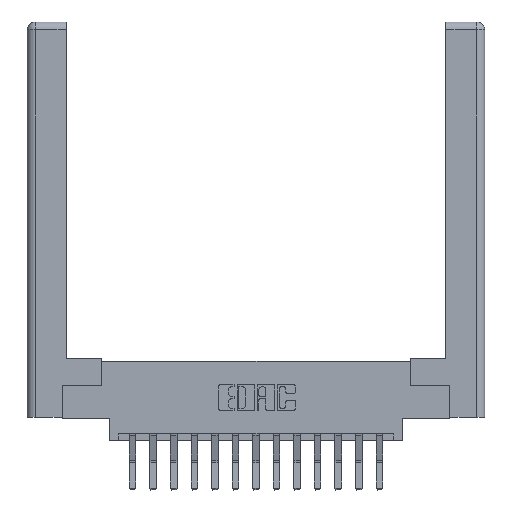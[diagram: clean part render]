
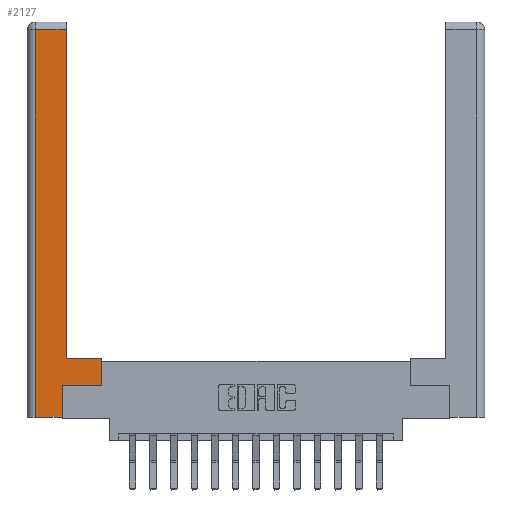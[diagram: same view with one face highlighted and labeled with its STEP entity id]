
A CAD part, top view. The second image highlights one B-rep face of the part: STEP entity #2127.
In plain terms, the highlighted planar face has unit normal (0, 0, 1).
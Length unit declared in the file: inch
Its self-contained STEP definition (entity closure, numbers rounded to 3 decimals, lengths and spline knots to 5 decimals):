
#1 = VECTOR ( 'NONE', #6524, 39.37008 ) ;
#176 = LINE ( 'NONE', #9322, #4261 ) ;
#615 = VERTEX_POINT ( 'NONE', #15131 ) ;
#640 = EDGE_CURVE ( 'NONE', #4127, #615, #4066, .T. ) ;
#830 = ORIENTED_EDGE ( 'NONE', *, *, #15073, .T. ) ;
#904 = CARTESIAN_POINT ( 'NONE',  ( 0., 0., 0. ) ) ;
#1306 = DIRECTION ( 'NONE',  ( 1., 0., 0. ) ) ;
#1787 = LINE ( 'NONE', #5879, #7243 ) ;
#2127 = ADVANCED_FACE ( 'NONE', ( #13701 ), #5015, .F. ) ;
#2202 = EDGE_CURVE ( 'NONE', #4471, #12927, #1787, .T. ) ;
#2537 = EDGE_LOOP ( 'NONE', ( #14064, #10161, #830, #11777, #7484, #6974, #5927, #4279 ) ) ;
#2657 = AXIS2_PLACEMENT_3D ( 'NONE', #904, #6328, #9095 ) ;
#2907 = VERTEX_POINT ( 'NONE', #4724 ) ;
#3094 = DIRECTION ( 'NONE',  ( -1., 0., 0. ) ) ;
#3812 = CARTESIAN_POINT ( 'NONE',  ( 0.265, 0., 0. ) ) ;
#4066 = LINE ( 'NONE', #14343, #1 ) ;
#4127 = VERTEX_POINT ( 'NONE', #9582 ) ;
#4261 = VECTOR ( 'NONE', #5508, 39.37008 ) ;
#4279 = ORIENTED_EDGE ( 'NONE', *, *, #16211, .T. ) ;
#4471 = VERTEX_POINT ( 'NONE', #13369 ) ;
#4724 = CARTESIAN_POINT ( 'NONE',  ( 0.565, 0.245, 0. ) ) ;
#4844 = DIRECTION ( 'NONE',  ( -1., 0., 0. ) ) ;
#5015 = PLANE ( 'NONE',  #2657 ) ;
#5061 = CARTESIAN_POINT ( 'NONE',  ( 0.0615, 2.94, 0. ) ) ;
#5339 = VECTOR ( 'NONE', #8675, 39.37008 ) ;
#5508 = DIRECTION ( 'NONE',  ( 0., 1., 0. ) ) ;
#5879 = CARTESIAN_POINT ( 'NONE',  ( 0.295, 3., 0. ) ) ;
#5902 = VECTOR ( 'NONE', #7099, 39.37008 ) ;
#5927 = ORIENTED_EDGE ( 'NONE', *, *, #5997, .T. ) ;
#5997 = EDGE_CURVE ( 'NONE', #2907, #6063, #176, .T. ) ;
#6063 = VERTEX_POINT ( 'NONE', #10544 ) ;
#6232 = CARTESIAN_POINT ( 'NONE',  ( 0.0615, 0., 0. ) ) ;
#6328 = DIRECTION ( 'NONE',  ( 0., 0., -1. ) ) ;
#6524 = DIRECTION ( 'NONE',  ( 0., 1., 0. ) ) ;
#6561 = VERTEX_POINT ( 'NONE', #5061 ) ;
#6716 = VECTOR ( 'NONE', #3094, 39.37008 ) ;
#6974 = ORIENTED_EDGE ( 'NONE', *, *, #9352, .T. ) ;
#7099 = DIRECTION ( 'NONE',  ( 0., -1., 0. ) ) ;
#7243 = VECTOR ( 'NONE', #9892, 39.37008 ) ;
#7256 = CARTESIAN_POINT ( 'NONE',  ( 0.565, 0.245, 0. ) ) ;
#7484 = ORIENTED_EDGE ( 'NONE', *, *, #640, .T. ) ;
#8583 = LINE ( 'NONE', #12562, #8961 ) ;
#8664 = VECTOR ( 'NONE', #1306, 39.37008 ) ;
#8675 = DIRECTION ( 'NONE',  ( 1., 0., 0. ) ) ;
#8795 = LINE ( 'NONE', #7256, #5339 ) ;
#8961 = VECTOR ( 'NONE', #4844, 39.37008 ) ;
#9095 = DIRECTION ( 'NONE',  ( -1., 0., 0. ) ) ;
#9322 = CARTESIAN_POINT ( 'NONE',  ( 0.565, 0.45, 0. ) ) ;
#9337 = LINE ( 'NONE', #10840, #5902 ) ;
#9352 = EDGE_CURVE ( 'NONE', #615, #2907, #8795, .T. ) ;
#9582 = CARTESIAN_POINT ( 'NONE',  ( 0.265, 0., 0. ) ) ;
#9892 = DIRECTION ( 'NONE',  ( 0., 1., 0. ) ) ;
#10161 = ORIENTED_EDGE ( 'NONE', *, *, #13758, .T. ) ;
#10499 = EDGE_CURVE ( 'NONE', #13332, #4127, #12892, .T. ) ;
#10544 = CARTESIAN_POINT ( 'NONE',  ( 0.565, 0.45, 0. ) ) ;
#10574 = LINE ( 'NONE', #13539, #6716 ) ;
#10840 = CARTESIAN_POINT ( 'NONE',  ( 0.0615, 0., 0. ) ) ;
#11777 = ORIENTED_EDGE ( 'NONE', *, *, #10499, .T. ) ;
#11831 = CARTESIAN_POINT ( 'NONE',  ( 0.295, 2.94, 0. ) ) ;
#12562 = CARTESIAN_POINT ( 'NONE',  ( 0.0615, 2.94, 0. ) ) ;
#12892 = LINE ( 'NONE', #3812, #8664 ) ;
#12927 = VERTEX_POINT ( 'NONE', #11831 ) ;
#13332 = VERTEX_POINT ( 'NONE', #6232 ) ;
#13369 = CARTESIAN_POINT ( 'NONE',  ( 0.295, 0.45, 0. ) ) ;
#13539 = CARTESIAN_POINT ( 'NONE',  ( 0.295, 0.45, 0. ) ) ;
#13701 = FACE_OUTER_BOUND ( 'NONE', #2537, .T. ) ;
#13758 = EDGE_CURVE ( 'NONE', #12927, #6561, #8583, .T. ) ;
#14064 = ORIENTED_EDGE ( 'NONE', *, *, #2202, .T. ) ;
#14343 = CARTESIAN_POINT ( 'NONE',  ( 0.265, 0.245, 0. ) ) ;
#15073 = EDGE_CURVE ( 'NONE', #6561, #13332, #9337, .T. ) ;
#15131 = CARTESIAN_POINT ( 'NONE',  ( 0.265, 0.245, 0. ) ) ;
#16211 = EDGE_CURVE ( 'NONE', #6063, #4471, #10574, .T. ) ;
